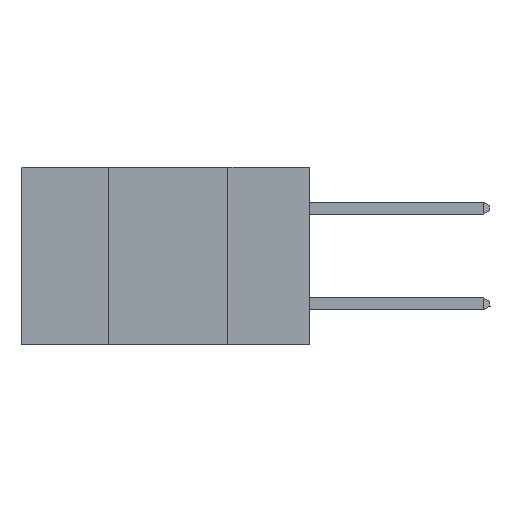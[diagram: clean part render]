
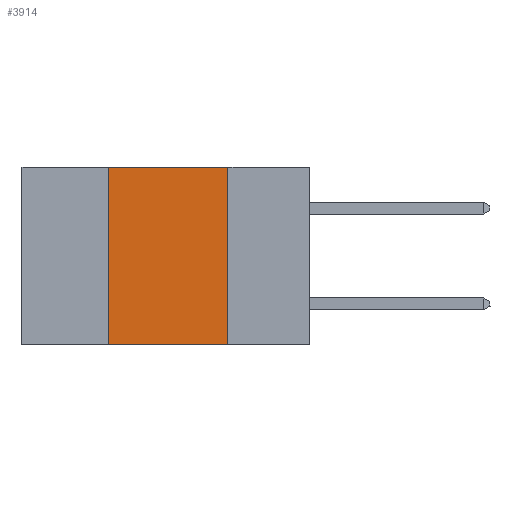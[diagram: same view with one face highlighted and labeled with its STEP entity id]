
A CAD part, left-side view. The second image highlights one B-rep face of the part: STEP entity #3914.
In plain terms, the highlighted planar face has unit normal (-1, 0, 0).
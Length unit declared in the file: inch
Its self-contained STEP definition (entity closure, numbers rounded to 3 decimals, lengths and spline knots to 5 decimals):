
#640 = EDGE_LOOP ( 'NONE', ( #11987, #7928, #10970, #18529 ) ) ;
#757 = LINE ( 'NONE', #14811, #15304 ) ;
#1165 = EDGE_CURVE ( 'NONE', #2510, #10913, #15527, .T. ) ;
#1545 = CARTESIAN_POINT ( 'NONE',  ( 0., 0.17, -0.37 ) ) ;
#1807 = VERTEX_POINT ( 'NONE', #1545 ) ;
#2069 = DIRECTION ( 'NONE',  ( 0., 0., -1. ) ) ;
#2447 = FACE_OUTER_BOUND ( 'NONE', #640, .T. ) ;
#2510 = VERTEX_POINT ( 'NONE', #18103 ) ;
#3914 = ADVANCED_FACE ( 'NONE', ( #2447 ), #9611, .F. ) ;
#4226 = DIRECTION ( 'NONE',  ( 0., -1., 0. ) ) ;
#4683 = VECTOR ( 'NONE', #18434, 39.37008 ) ;
#5790 = CARTESIAN_POINT ( 'NONE',  ( 0., 0.42, -0.37 ) ) ;
#6233 = AXIS2_PLACEMENT_3D ( 'NONE', #17820, #18089, #2069 ) ;
#7111 = EDGE_CURVE ( 'NONE', #9080, #1807, #11394, .T. ) ;
#7928 = ORIENTED_EDGE ( 'NONE', *, *, #1165, .F. ) ;
#8205 = VECTOR ( 'NONE', #4226, 39.37008 ) ;
#9080 = VERTEX_POINT ( 'NONE', #5790 ) ;
#9514 = DIRECTION ( 'NONE',  ( 0., 0., -1. ) ) ;
#9611 = PLANE ( 'NONE',  #6233 ) ;
#10913 = VERTEX_POINT ( 'NONE', #17814 ) ;
#10970 = ORIENTED_EDGE ( 'NONE', *, *, #17412, .F. ) ;
#11394 = LINE ( 'NONE', #12074, #8205 ) ;
#11668 = VECTOR ( 'NONE', #9514, 39.37008 ) ;
#11987 = ORIENTED_EDGE ( 'NONE', *, *, #13476, .F. ) ;
#12074 = CARTESIAN_POINT ( 'NONE',  ( 0., 0.6, -0.37 ) ) ;
#12429 = CARTESIAN_POINT ( 'NONE',  ( 0., 0.6, 0. ) ) ;
#13476 = EDGE_CURVE ( 'NONE', #10913, #1807, #18446, .T. ) ;
#14811 = CARTESIAN_POINT ( 'NONE',  ( 0., 0.42, 0. ) ) ;
#15304 = VECTOR ( 'NONE', #17916, 39.37008 ) ;
#15527 = LINE ( 'NONE', #12429, #4683 ) ;
#17412 = EDGE_CURVE ( 'NONE', #9080, #2510, #757, .T. ) ;
#17814 = CARTESIAN_POINT ( 'NONE',  ( 0., 0.17, 0. ) ) ;
#17820 = CARTESIAN_POINT ( 'NONE',  ( 0., 0.6, 0. ) ) ;
#17916 = DIRECTION ( 'NONE',  ( 0., 0., 1. ) ) ;
#18087 = CARTESIAN_POINT ( 'NONE',  ( 0., 0.17, 0. ) ) ;
#18089 = DIRECTION ( 'NONE',  ( 1., 0., 0. ) ) ;
#18103 = CARTESIAN_POINT ( 'NONE',  ( 0., 0.42, 0. ) ) ;
#18434 = DIRECTION ( 'NONE',  ( 0., -1., 0. ) ) ;
#18446 = LINE ( 'NONE', #18087, #11668 ) ;
#18529 = ORIENTED_EDGE ( 'NONE', *, *, #7111, .T. ) ;
